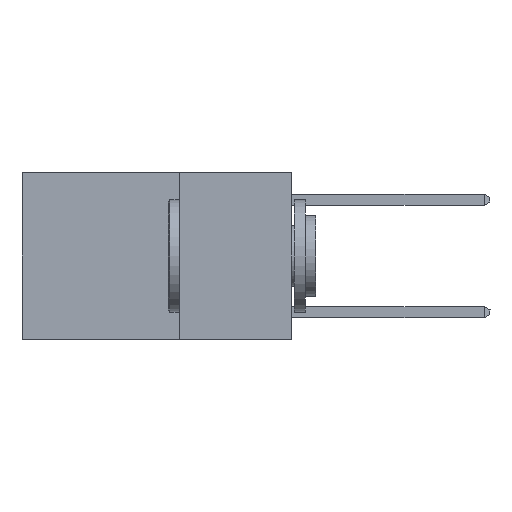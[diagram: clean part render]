
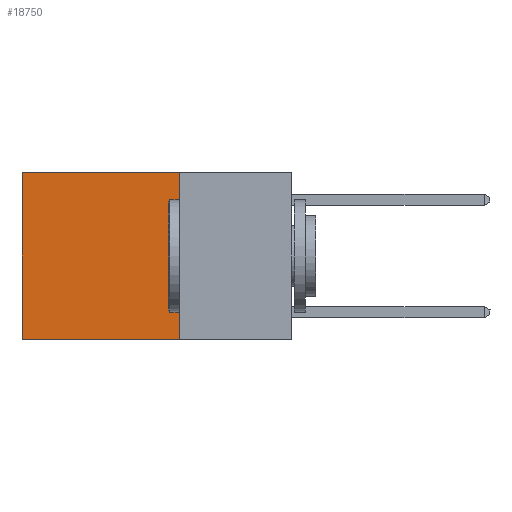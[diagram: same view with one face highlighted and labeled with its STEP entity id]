
A CAD part, left-side view. The second image highlights one B-rep face of the part: STEP entity #18750.
In plain terms, the highlighted planar face has unit normal (-1, 0, 0).
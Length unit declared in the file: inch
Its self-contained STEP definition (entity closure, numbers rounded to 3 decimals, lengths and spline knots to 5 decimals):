
#267 = CARTESIAN_POINT ( 'NONE',  ( 0.2625, 0.25, 0. ) ) ;
#1355 = VERTEX_POINT ( 'NONE', #9816 ) ;
#1476 = ORIENTED_EDGE ( 'NONE', *, *, #8804, .F. ) ;
#2657 = EDGE_CURVE ( 'NONE', #16187, #1355, #6762, .T. ) ;
#3592 = CARTESIAN_POINT ( 'NONE',  ( 0.2625, 0.6, 0. ) ) ;
#3770 = LINE ( 'NONE', #4763, #12677 ) ;
#4530 = EDGE_CURVE ( 'NONE', #7850, #1355, #3770, .T. ) ;
#4763 = CARTESIAN_POINT ( 'NONE',  ( 0.2625, 0.25, -0.37 ) ) ;
#4894 = DIRECTION ( 'NONE',  ( 0., 0., -1. ) ) ;
#5181 = EDGE_LOOP ( 'NONE', ( #20726, #18105, #1476, #8498 ) ) ;
#5481 = LINE ( 'NONE', #267, #18283 ) ;
#6458 = DIRECTION ( 'NONE',  ( 0., 1., 0. ) ) ;
#6762 = LINE ( 'NONE', #6998, #14952 ) ;
#6998 = CARTESIAN_POINT ( 'NONE',  ( 0.2625, 0.6, 0. ) ) ;
#7850 = VERTEX_POINT ( 'NONE', #17895 ) ;
#8267 = VECTOR ( 'NONE', #19218, 39.37008 ) ;
#8498 = ORIENTED_EDGE ( 'NONE', *, *, #14646, .T. ) ;
#8804 = EDGE_CURVE ( 'NONE', #11942, #7850, #5481, .T. ) ;
#9816 = CARTESIAN_POINT ( 'NONE',  ( 0.2625, 0.6, -0.37 ) ) ;
#10397 = DIRECTION ( 'NONE',  ( 0., 0., -1. ) ) ;
#10515 = DIRECTION ( 'NONE',  ( 0., 0., -1. ) ) ;
#11586 = CARTESIAN_POINT ( 'NONE',  ( 0.2625, 0.25, 0. ) ) ;
#11825 = FACE_OUTER_BOUND ( 'NONE', #5181, .T. ) ;
#11942 = VERTEX_POINT ( 'NONE', #18980 ) ;
#12677 = VECTOR ( 'NONE', #6458, 39.37008 ) ;
#13195 = PLANE ( 'NONE',  #20552 ) ;
#14646 = EDGE_CURVE ( 'NONE', #11942, #16187, #20645, .T. ) ;
#14763 = DIRECTION ( 'NONE',  ( 1., 0., 0. ) ) ;
#14952 = VECTOR ( 'NONE', #10397, 39.37008 ) ;
#16187 = VERTEX_POINT ( 'NONE', #3592 ) ;
#17895 = CARTESIAN_POINT ( 'NONE',  ( 0.2625, 0.25, -0.37 ) ) ;
#18105 = ORIENTED_EDGE ( 'NONE', *, *, #4530, .F. ) ;
#18283 = VECTOR ( 'NONE', #10515, 39.37008 ) ;
#18750 = ADVANCED_FACE ( 'NONE', ( #11825 ), #13195, .F. ) ;
#18980 = CARTESIAN_POINT ( 'NONE',  ( 0.2625, 0.25, 0. ) ) ;
#19218 = DIRECTION ( 'NONE',  ( 0., 1., 0. ) ) ;
#20552 = AXIS2_PLACEMENT_3D ( 'NONE', #11586, #14763, #4894 ) ;
#20645 = LINE ( 'NONE', #20650, #8267 ) ;
#20650 = CARTESIAN_POINT ( 'NONE',  ( 0.2625, 0.25, 0. ) ) ;
#20726 = ORIENTED_EDGE ( 'NONE', *, *, #2657, .T. ) ;
